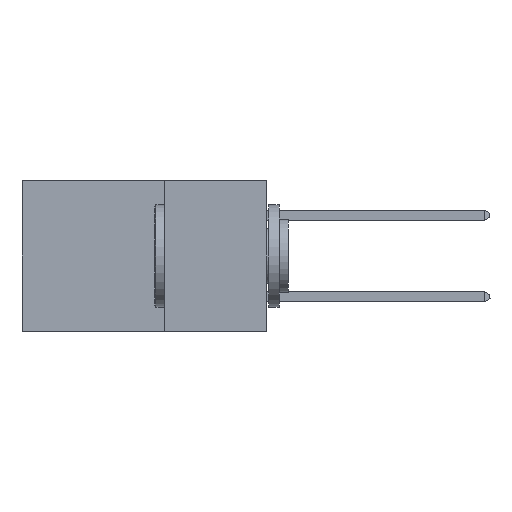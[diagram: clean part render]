
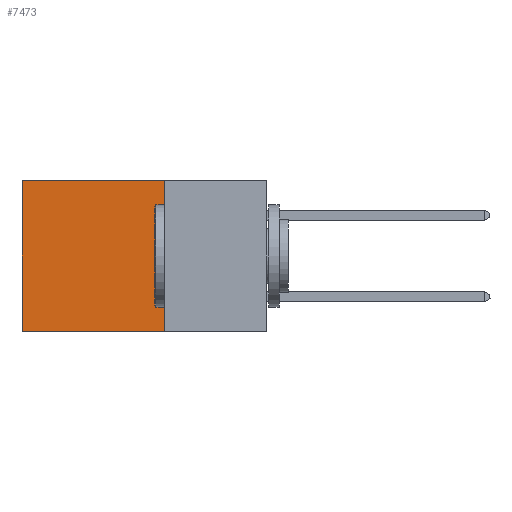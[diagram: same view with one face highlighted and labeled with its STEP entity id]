
A CAD part, left-side view. The second image highlights one B-rep face of the part: STEP entity #7473.
In plain terms, the highlighted planar face has unit normal (-1, 0, 0).
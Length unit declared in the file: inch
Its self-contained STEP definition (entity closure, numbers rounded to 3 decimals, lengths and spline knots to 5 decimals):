
#1081 = DIRECTION ( 'NONE',  ( 0., 0., -1. ) ) ;
#3591 = VERTEX_POINT ( 'NONE', #28786 ) ;
#6786 = CARTESIAN_POINT ( 'NONE',  ( 0.2875, 0.6, 0. ) ) ;
#7473 = ADVANCED_FACE ( 'NONE', ( #24403 ), #24915, .F. ) ;
#8187 = CARTESIAN_POINT ( 'NONE',  ( 0.2875, 0.25, 0. ) ) ;
#11146 = CARTESIAN_POINT ( 'NONE',  ( 0.2875, 0.6, -0.37 ) ) ;
#11147 = CARTESIAN_POINT ( 'NONE',  ( 0.2875, 0.6, 0. ) ) ;
#11476 = LINE ( 'NONE', #23058, #29556 ) ;
#12651 = DIRECTION ( 'NONE',  ( 0., 1., 0. ) ) ;
#13245 = ORIENTED_EDGE ( 'NONE', *, *, #20105, .F. ) ;
#19662 = AXIS2_PLACEMENT_3D ( 'NONE', #40281, #28847, #36481 ) ;
#20105 = EDGE_CURVE ( 'NONE', #24158, #3591, #34069, .T. ) ;
#20208 = EDGE_CURVE ( 'NONE', #3591, #43287, #11476, .T. ) ;
#20991 = VECTOR ( 'NONE', #29149, 39.37008 ) ;
#21536 = ORIENTED_EDGE ( 'NONE', *, *, #23448, .T. ) ;
#23038 = DIRECTION ( 'NONE',  ( 0., 1., 0. ) ) ;
#23058 = CARTESIAN_POINT ( 'NONE',  ( 0.2875, 0.25, -0.37 ) ) ;
#23448 = EDGE_CURVE ( 'NONE', #24158, #42222, #43519, .T. ) ;
#23821 = EDGE_CURVE ( 'NONE', #42222, #43287, #39545, .T. ) ;
#24158 = VERTEX_POINT ( 'NONE', #45125 ) ;
#24403 = FACE_OUTER_BOUND ( 'NONE', #29991, .T. ) ;
#24915 = PLANE ( 'NONE',  #19662 ) ;
#27758 = VECTOR ( 'NONE', #23038, 39.37008 ) ;
#28786 = CARTESIAN_POINT ( 'NONE',  ( 0.2875, 0.25, -0.37 ) ) ;
#28847 = DIRECTION ( 'NONE',  ( 1., 0., 0. ) ) ;
#29149 = DIRECTION ( 'NONE',  ( 0., 0., -1. ) ) ;
#29556 = VECTOR ( 'NONE', #12651, 39.37008 ) ;
#29991 = EDGE_LOOP ( 'NONE', ( #37481, #41147, #13245, #21536 ) ) ;
#34069 = LINE ( 'NONE', #8187, #38602 ) ;
#36481 = DIRECTION ( 'NONE',  ( 0., 0., -1. ) ) ;
#37481 = ORIENTED_EDGE ( 'NONE', *, *, #23821, .T. ) ;
#37768 = CARTESIAN_POINT ( 'NONE',  ( 0.2875, 0.25, 0. ) ) ;
#38602 = VECTOR ( 'NONE', #1081, 39.37008 ) ;
#39545 = LINE ( 'NONE', #11147, #20991 ) ;
#40281 = CARTESIAN_POINT ( 'NONE',  ( 0.2875, 0.25, 0. ) ) ;
#41147 = ORIENTED_EDGE ( 'NONE', *, *, #20208, .F. ) ;
#42222 = VERTEX_POINT ( 'NONE', #6786 ) ;
#43287 = VERTEX_POINT ( 'NONE', #11146 ) ;
#43519 = LINE ( 'NONE', #37768, #27758 ) ;
#45125 = CARTESIAN_POINT ( 'NONE',  ( 0.2875, 0.25, 0. ) ) ;
